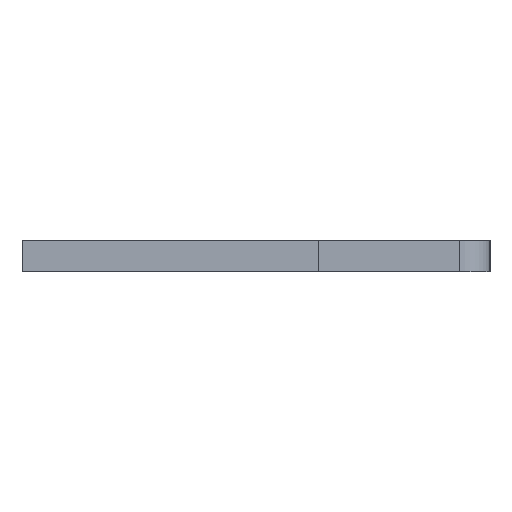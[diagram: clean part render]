
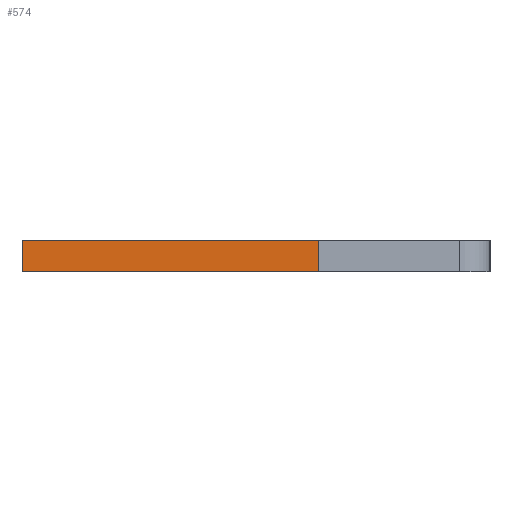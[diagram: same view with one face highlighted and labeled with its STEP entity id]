
A CAD part, left-side view. The second image highlights one B-rep face of the part: STEP entity #574.
In plain terms, the highlighted face is planar.
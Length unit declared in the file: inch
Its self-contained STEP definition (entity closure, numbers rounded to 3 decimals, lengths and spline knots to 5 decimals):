
#3 = EDGE_CURVE ( 'NONE', #250, #1968, #952, .T. ) ;
#112 = EDGE_CURVE ( 'NONE', #1947, #250, #1945, .T. ) ;
#126 = VECTOR ( 'NONE', #243, 39.37008 ) ;
#148 = CARTESIAN_POINT ( 'NONE',  ( 0.01, 0.15, -0.04 ) ) ;
#172 = CARTESIAN_POINT ( 'NONE',  ( 0.01, -0.04, -0.04 ) ) ;
#243 = DIRECTION ( 'NONE',  ( -1., 0., 0. ) ) ;
#250 = VERTEX_POINT ( 'NONE', #1465 ) ;
#548 = DIRECTION ( 'NONE',  ( 0., 0., 1. ) ) ;
#574 = ADVANCED_FACE ( 'NONE', ( #981 ), #1705, .F. ) ;
#614 = DIRECTION ( 'NONE',  ( 1., 0., 0. ) ) ;
#699 = CARTESIAN_POINT ( 'NONE',  ( 0.01, 0.15, -0.04 ) ) ;
#876 = DIRECTION ( 'NONE',  ( 0., 1., 0. ) ) ;
#897 = LINE ( 'NONE', #1657, #1674 ) ;
#952 = LINE ( 'NONE', #1011, #126 ) ;
#957 = DIRECTION ( 'NONE',  ( -1., 0., 0. ) ) ;
#981 = FACE_OUTER_BOUND ( 'NONE', #1948, .T. ) ;
#1011 = CARTESIAN_POINT ( 'NONE',  ( 0.01, 0.15, -0.04 ) ) ;
#1119 = EDGE_CURVE ( 'NONE', #1947, #1552, #1124, .T. ) ;
#1124 = LINE ( 'NONE', #172, #1366 ) ;
#1330 = CARTESIAN_POINT ( 'NONE',  ( -0.01, 0.15, -0.04 ) ) ;
#1366 = VECTOR ( 'NONE', #957, 39.37008 ) ;
#1465 = CARTESIAN_POINT ( 'NONE',  ( 0.01, 0.15, -0.04 ) ) ;
#1498 = CARTESIAN_POINT ( 'NONE',  ( 0.01, -0.04, -0.04 ) ) ;
#1552 = VERTEX_POINT ( 'NONE', #1625 ) ;
#1590 = AXIS2_PLACEMENT_3D ( 'NONE', #148, #548, #614 ) ;
#1619 = VECTOR ( 'NONE', #1813, 39.37008 ) ;
#1625 = CARTESIAN_POINT ( 'NONE',  ( -0.01, -0.04, -0.04 ) ) ;
#1657 = CARTESIAN_POINT ( 'NONE',  ( -0.01, 0.15, -0.04 ) ) ;
#1674 = VECTOR ( 'NONE', #876, 39.37008 ) ;
#1705 = PLANE ( 'NONE',  #1590 ) ;
#1706 = ORIENTED_EDGE ( 'NONE', *, *, #1806, .T. ) ;
#1713 = ORIENTED_EDGE ( 'NONE', *, *, #1119, .T. ) ;
#1806 = EDGE_CURVE ( 'NONE', #1552, #1968, #897, .T. ) ;
#1813 = DIRECTION ( 'NONE',  ( 0., 1., 0. ) ) ;
#1880 = ORIENTED_EDGE ( 'NONE', *, *, #112, .F. ) ;
#1945 = LINE ( 'NONE', #699, #1619 ) ;
#1947 = VERTEX_POINT ( 'NONE', #1498 ) ;
#1948 = EDGE_LOOP ( 'NONE', ( #1706, #1999, #1880, #1713 ) ) ;
#1968 = VERTEX_POINT ( 'NONE', #1330 ) ;
#1999 = ORIENTED_EDGE ( 'NONE', *, *, #3, .F. ) ;
